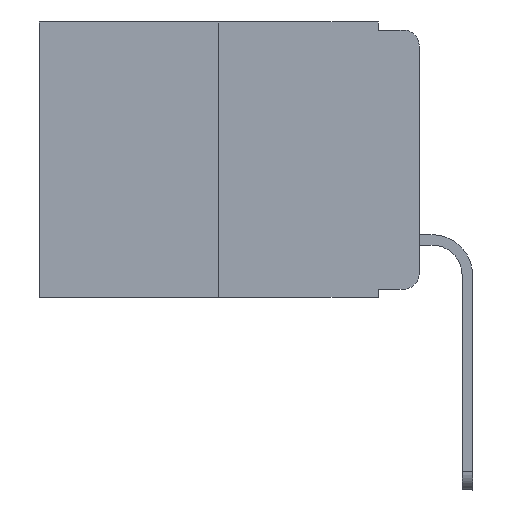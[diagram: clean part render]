
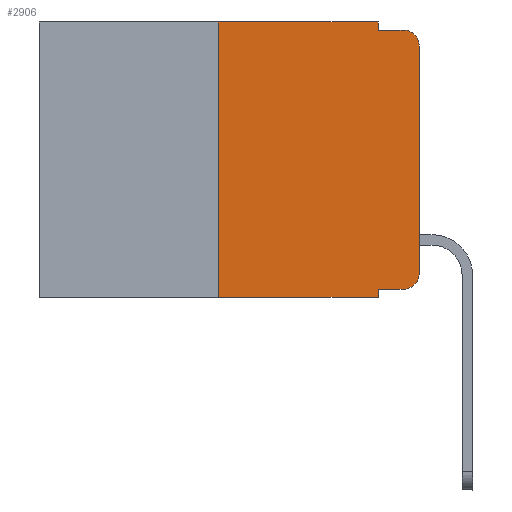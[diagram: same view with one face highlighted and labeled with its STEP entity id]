
A CAD part, left-side view. The second image highlights one B-rep face of the part: STEP entity #2906.
In plain terms, the highlighted planar face has unit normal (-1, 0, 0).
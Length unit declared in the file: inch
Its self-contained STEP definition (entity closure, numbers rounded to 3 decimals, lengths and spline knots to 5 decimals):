
#106 = DIRECTION ( 'NONE',  ( 0., 0., -1. ) ) ;
#576 = PLANE ( 'NONE',  #6854 ) ;
#692 = CARTESIAN_POINT ( 'NONE',  ( 0., 0.25, 0. ) ) ;
#712 = EDGE_CURVE ( 'NONE', #8329, #9851, #12789, .T. ) ;
#732 = ORIENTED_EDGE ( 'NONE', *, *, #7134, .F. ) ;
#918 = EDGE_CURVE ( 'NONE', #13991, #3545, #3198, .T. ) ;
#1179 = LINE ( 'NONE', #10437, #8197 ) ;
#1406 = CARTESIAN_POINT ( 'NONE',  ( 0., 0.473, -0.343 ) ) ;
#1503 = ORIENTED_EDGE ( 'NONE', *, *, #6727, .T. ) ;
#1506 = CARTESIAN_POINT ( 'NONE',  ( 0., 0.051, -0.333 ) ) ;
#1526 = CARTESIAN_POINT ( 'NONE',  ( 0., 0.051, 0. ) ) ;
#1646 = ORIENTED_EDGE ( 'NONE', *, *, #4153, .F. ) ;
#2310 = DIRECTION ( 'NONE',  ( 0., 0., 1. ) ) ;
#2665 = DIRECTION ( 'NONE',  ( -1., 0., 0. ) ) ;
#2873 = EDGE_CURVE ( 'NONE', #10910, #8697, #3661, .T. ) ;
#2906 = ADVANCED_FACE ( 'NONE', ( #6300 ), #576, .F. ) ;
#2928 = ORIENTED_EDGE ( 'NONE', *, *, #14080, .T. ) ;
#3059 = ORIENTED_EDGE ( 'NONE', *, *, #3975, .F. ) ;
#3198 = CIRCLE ( 'NONE', #5851, 0.02 ) ;
#3507 = ORIENTED_EDGE ( 'NONE', *, *, #712, .F. ) ;
#3545 = VERTEX_POINT ( 'NONE', #5301 ) ;
#3661 = LINE ( 'NONE', #1406, #6369 ) ;
#3850 = CARTESIAN_POINT ( 'NONE',  ( 0., 0., -0.03 ) ) ;
#3891 = DIRECTION ( 'NONE',  ( 1., 0., 0. ) ) ;
#3975 = EDGE_CURVE ( 'NONE', #9851, #10968, #1179, .T. ) ;
#4153 = EDGE_CURVE ( 'NONE', #8120, #8329, #11919, .T. ) ;
#4423 = VECTOR ( 'NONE', #106, 39.37008 ) ;
#4559 = CARTESIAN_POINT ( 'NONE',  ( 0., 0.051, 0. ) ) ;
#4968 = CARTESIAN_POINT ( 'NONE',  ( 0., 0.473, 0. ) ) ;
#4971 = DIRECTION ( 'NONE',  ( 0., -1., 0. ) ) ;
#5301 = CARTESIAN_POINT ( 'NONE',  ( 0., 0., -0.313 ) ) ;
#5393 = AXIS2_PLACEMENT_3D ( 'NONE', #13434, #9407, #7010 ) ;
#5447 = LINE ( 'NONE', #7843, #7680 ) ;
#5808 = CARTESIAN_POINT ( 'NONE',  ( 0., 0.051, -0.01 ) ) ;
#5851 = AXIS2_PLACEMENT_3D ( 'NONE', #14127, #2665, #8588 ) ;
#5862 = DIRECTION ( 'NONE',  ( 0., -1., 0. ) ) ;
#5947 = ORIENTED_EDGE ( 'NONE', *, *, #10777, .F. ) ;
#6050 = LINE ( 'NONE', #11590, #8915 ) ;
#6203 = DIRECTION ( 'NONE',  ( 0., 0., -1. ) ) ;
#6300 = FACE_OUTER_BOUND ( 'NONE', #13955, .T. ) ;
#6369 = VECTOR ( 'NONE', #6980, 39.37008 ) ;
#6727 = EDGE_CURVE ( 'NONE', #3545, #7067, #14214, .T. ) ;
#6854 = AXIS2_PLACEMENT_3D ( 'NONE', #4968, #3891, #14301 ) ;
#6861 = ORIENTED_EDGE ( 'NONE', *, *, #918, .T. ) ;
#6980 = DIRECTION ( 'NONE',  ( 0., -1., 0. ) ) ;
#7010 = DIRECTION ( 'NONE',  ( 0., 0., -1. ) ) ;
#7054 = CARTESIAN_POINT ( 'NONE',  ( 0., 0.25, 0. ) ) ;
#7067 = VERTEX_POINT ( 'NONE', #3850 ) ;
#7134 = EDGE_CURVE ( 'NONE', #13001, #8697, #6050, .T. ) ;
#7406 = DIRECTION ( 'NONE',  ( 0., 0., 1. ) ) ;
#7680 = VECTOR ( 'NONE', #14644, 39.37008 ) ;
#7843 = CARTESIAN_POINT ( 'NONE',  ( 0., 0.051, -0.333 ) ) ;
#8018 = CIRCLE ( 'NONE', #5393, 0.02 ) ;
#8069 = ORIENTED_EDGE ( 'NONE', *, *, #2873, .T. ) ;
#8114 = ORIENTED_EDGE ( 'NONE', *, *, #9850, .T. ) ;
#8120 = VERTEX_POINT ( 'NONE', #692 ) ;
#8197 = VECTOR ( 'NONE', #5862, 39.37008 ) ;
#8329 = VERTEX_POINT ( 'NONE', #1526 ) ;
#8588 = DIRECTION ( 'NONE',  ( 0., 0., -1. ) ) ;
#8697 = VERTEX_POINT ( 'NONE', #10081 ) ;
#8915 = VECTOR ( 'NONE', #6203, 39.37008 ) ;
#9407 = DIRECTION ( 'NONE',  ( -1., 0., 0. ) ) ;
#9850 = EDGE_CURVE ( 'NONE', #7067, #10968, #8018, .T. ) ;
#9851 = VERTEX_POINT ( 'NONE', #5808 ) ;
#10081 = CARTESIAN_POINT ( 'NONE',  ( 0., 0.051, -0.343 ) ) ;
#10437 = CARTESIAN_POINT ( 'NONE',  ( 0., 0.051, -0.01 ) ) ;
#10561 = CARTESIAN_POINT ( 'NONE',  ( 0., 0.25, -0.343 ) ) ;
#10675 = VECTOR ( 'NONE', #2310, 39.37008 ) ;
#10777 = EDGE_CURVE ( 'NONE', #10910, #8120, #12733, .T. ) ;
#10910 = VERTEX_POINT ( 'NONE', #10561 ) ;
#10968 = VERTEX_POINT ( 'NONE', #13524 ) ;
#11590 = CARTESIAN_POINT ( 'NONE',  ( 0., 0.051, 0. ) ) ;
#11684 = CARTESIAN_POINT ( 'NONE',  ( 0., 0., 0. ) ) ;
#11919 = LINE ( 'NONE', #13036, #12994 ) ;
#12406 = CARTESIAN_POINT ( 'NONE',  ( 0., 0.02, -0.333 ) ) ;
#12590 = VECTOR ( 'NONE', #7406, 39.37008 ) ;
#12733 = LINE ( 'NONE', #7054, #10675 ) ;
#12789 = LINE ( 'NONE', #4559, #4423 ) ;
#12994 = VECTOR ( 'NONE', #4971, 39.37008 ) ;
#13001 = VERTEX_POINT ( 'NONE', #1506 ) ;
#13036 = CARTESIAN_POINT ( 'NONE',  ( 0., 0.473, 0. ) ) ;
#13434 = CARTESIAN_POINT ( 'NONE',  ( 0., 0.02, -0.03 ) ) ;
#13524 = CARTESIAN_POINT ( 'NONE',  ( 0., 0.02, -0.01 ) ) ;
#13955 = EDGE_LOOP ( 'NONE', ( #1503, #8114, #3059, #3507, #1646, #5947, #8069, #732, #2928, #6861 ) ) ;
#13991 = VERTEX_POINT ( 'NONE', #12406 ) ;
#14080 = EDGE_CURVE ( 'NONE', #13001, #13991, #5447, .T. ) ;
#14127 = CARTESIAN_POINT ( 'NONE',  ( 0., 0.02, -0.313 ) ) ;
#14214 = LINE ( 'NONE', #11684, #12590 ) ;
#14301 = DIRECTION ( 'NONE',  ( 0., 0., -1. ) ) ;
#14644 = DIRECTION ( 'NONE',  ( 0., -1., 0. ) ) ;
